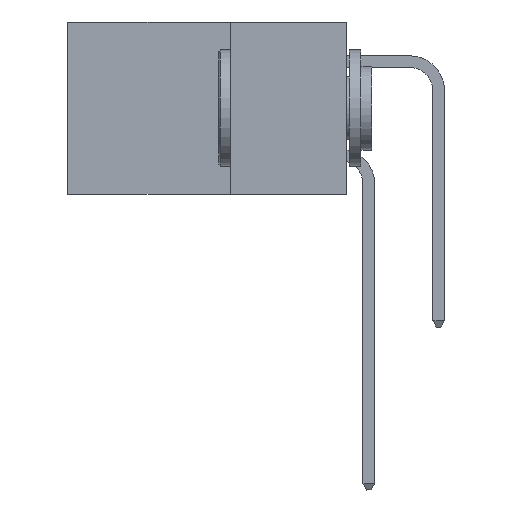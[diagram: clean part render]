
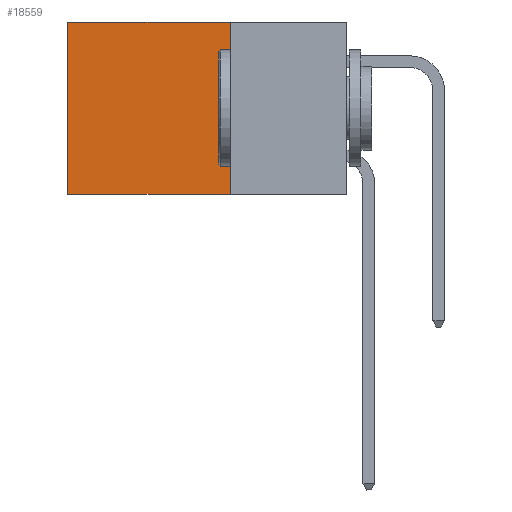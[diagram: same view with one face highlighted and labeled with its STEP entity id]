
A CAD part, left-side view. The second image highlights one B-rep face of the part: STEP entity #18559.
In plain terms, the highlighted planar face has unit normal (-1, 0, 0).
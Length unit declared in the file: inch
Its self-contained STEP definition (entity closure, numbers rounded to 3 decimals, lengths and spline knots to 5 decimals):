
#152 = ORIENTED_EDGE ( 'NONE', *, *, #25851, .T. ) ;
#158 = VECTOR ( 'NONE', #12653, 39.37008 ) ;
#412 = VECTOR ( 'NONE', #16387, 39.37008 ) ;
#1108 = VERTEX_POINT ( 'NONE', #13975 ) ;
#2432 = EDGE_LOOP ( 'NONE', ( #25465, #8524, #20835, #152 ) ) ;
#3255 = VERTEX_POINT ( 'NONE', #16701 ) ;
#4863 = CARTESIAN_POINT ( 'NONE',  ( 0.2875, 0.25, 0. ) ) ;
#5552 = VECTOR ( 'NONE', #28119, 39.37008 ) ;
#5602 = CARTESIAN_POINT ( 'NONE',  ( 0.2875, 0.25, 0. ) ) ;
#6298 = LINE ( 'NONE', #4863, #5552 ) ;
#6365 = LINE ( 'NONE', #5602, #158 ) ;
#6786 = FACE_OUTER_BOUND ( 'NONE', #2432, .T. ) ;
#7335 = PLANE ( 'NONE',  #15303 ) ;
#8524 = ORIENTED_EDGE ( 'NONE', *, *, #15156, .F. ) ;
#9671 = DIRECTION ( 'NONE',  ( 1., 0., 0. ) ) ;
#10476 = CARTESIAN_POINT ( 'NONE',  ( 0.2875, 0.25, -0.37 ) ) ;
#10769 = VERTEX_POINT ( 'NONE', #16866 ) ;
#11721 = VERTEX_POINT ( 'NONE', #27527 ) ;
#12113 = VECTOR ( 'NONE', #15183, 39.37008 ) ;
#12653 = DIRECTION ( 'NONE',  ( 0., 0., -1. ) ) ;
#12837 = LINE ( 'NONE', #29797, #412 ) ;
#12856 = EDGE_CURVE ( 'NONE', #3255, #11721, #6365, .T. ) ;
#13975 = CARTESIAN_POINT ( 'NONE',  ( 0.2875, 0.6, 0. ) ) ;
#15156 = EDGE_CURVE ( 'NONE', #11721, #10769, #19066, .T. ) ;
#15183 = DIRECTION ( 'NONE',  ( 0., 1., 0. ) ) ;
#15303 = AXIS2_PLACEMENT_3D ( 'NONE', #23571, #9671, #25902 ) ;
#16387 = DIRECTION ( 'NONE',  ( 0., 0., -1. ) ) ;
#16701 = CARTESIAN_POINT ( 'NONE',  ( 0.2875, 0.25, 0. ) ) ;
#16866 = CARTESIAN_POINT ( 'NONE',  ( 0.2875, 0.6, -0.37 ) ) ;
#18559 = ADVANCED_FACE ( 'NONE', ( #6786 ), #7335, .F. ) ;
#19066 = LINE ( 'NONE', #10476, #12113 ) ;
#20835 = ORIENTED_EDGE ( 'NONE', *, *, #12856, .F. ) ;
#23571 = CARTESIAN_POINT ( 'NONE',  ( 0.2875, 0.25, 0. ) ) ;
#25465 = ORIENTED_EDGE ( 'NONE', *, *, #26515, .T. ) ;
#25851 = EDGE_CURVE ( 'NONE', #3255, #1108, #6298, .T. ) ;
#25902 = DIRECTION ( 'NONE',  ( 0., 0., -1. ) ) ;
#26515 = EDGE_CURVE ( 'NONE', #1108, #10769, #12837, .T. ) ;
#27527 = CARTESIAN_POINT ( 'NONE',  ( 0.2875, 0.25, -0.37 ) ) ;
#28119 = DIRECTION ( 'NONE',  ( 0., 1., 0. ) ) ;
#29797 = CARTESIAN_POINT ( 'NONE',  ( 0.2875, 0.6, 0. ) ) ;
